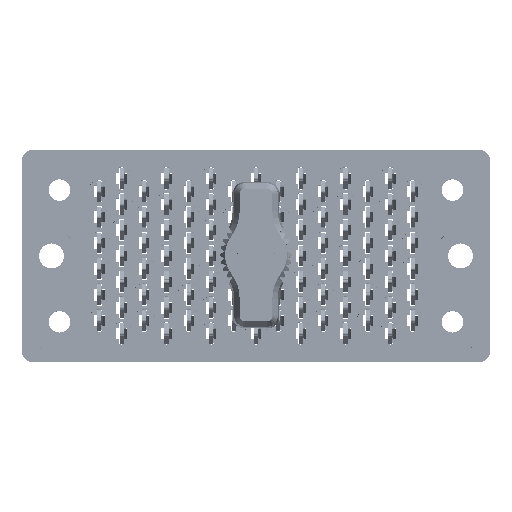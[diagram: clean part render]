
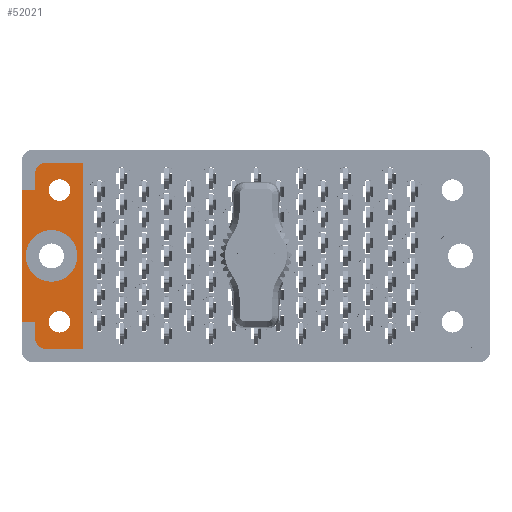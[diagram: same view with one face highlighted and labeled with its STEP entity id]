
A CAD part, top view. The second image highlights one B-rep face of the part: STEP entity #52021.
In plain terms, the highlighted planar face has unit normal (0, 0, 1).
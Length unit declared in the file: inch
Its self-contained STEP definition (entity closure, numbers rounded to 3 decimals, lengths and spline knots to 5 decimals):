
#267 = VECTOR ( 'NONE', #81808, 39.37008 ) ;
#488 = EDGE_CURVE ( 'NONE', #83931, #20014, #40906, .T. ) ;
#1366 = VERTEX_POINT ( 'NONE', #52308 ) ;
#2363 = AXIS2_PLACEMENT_3D ( 'NONE', #50024, #71200, #44172 ) ;
#2809 = ORIENTED_EDGE ( 'NONE', *, *, #488, .F. ) ;
#3448 = CARTESIAN_POINT ( 'NONE',  ( -1.1875, 0., -0.117 ) ) ;
#3648 = VERTEX_POINT ( 'NONE', #65361 ) ;
#3666 = EDGE_CURVE ( 'NONE', #20014, #83931, #4543, .T. ) ;
#4205 = ORIENTED_EDGE ( 'NONE', *, *, #11239, .F. ) ;
#4473 = EDGE_LOOP ( 'NONE', ( #41305, #84338, #61093, #54283, #52065, #55893, #63187, #67300, #24666, #56260 ) ) ;
#4543 = CIRCLE ( 'NONE', #33887, 0.0625 ) ;
#4942 = DIRECTION ( 'NONE',  ( 0., 0., 1. ) ) ;
#5032 = CIRCLE ( 'NONE', #50706, 0.062 ) ;
#5864 = CARTESIAN_POINT ( 'NONE',  ( -1.141, -0.3825, -0.117 ) ) ;
#6623 = EDGE_CURVE ( 'NONE', #80473, #18979, #70493, .T. ) ;
#7171 = CARTESIAN_POINT ( 'NONE',  ( -1.359, 0.617, -0.117 ) ) ;
#8485 = DIRECTION ( 'NONE',  ( 0., 0., 1. ) ) ;
#9338 = EDGE_CURVE ( 'NONE', #66660, #40700, #49050, .T. ) ;
#9568 = EDGE_CURVE ( 'NONE', #34214, #63157, #55380, .T. ) ;
#10014 = DIRECTION ( 'NONE',  ( 0., 0., 1. ) ) ;
#10477 = CARTESIAN_POINT ( 'NONE',  ( -1.2825, 0., -0.117 ) ) ;
#11239 = EDGE_CURVE ( 'NONE', #18979, #80473, #52926, .T. ) ;
#12429 = ORIENTED_EDGE ( 'NONE', *, *, #13034, .F. ) ;
#12678 = CARTESIAN_POINT ( 'NONE',  ( 0., -0.3825, -0.117 ) ) ;
#13034 = EDGE_CURVE ( 'NONE', #40700, #66660, #16687, .T. ) ;
#15766 = ORIENTED_EDGE ( 'NONE', *, *, #9338, .F. ) ;
#16687 = CIRCLE ( 'NONE', #18659, 0.0625 ) ;
#17314 = CARTESIAN_POINT ( 'NONE',  ( -1.005, 0.617, -0.117 ) ) ;
#17537 = CARTESIAN_POINT ( 'NONE',  ( -1.005, -0.54, -0.117 ) ) ;
#18172 = DIRECTION ( 'NONE',  ( 0., 1., 0. ) ) ;
#18659 = AXIS2_PLACEMENT_3D ( 'NONE', #79524, #4942, #59246 ) ;
#18979 = VERTEX_POINT ( 'NONE', #20722 ) ;
#19169 = DIRECTION ( 'NONE',  ( 0., -1., 0. ) ) ;
#19400 = EDGE_LOOP ( 'NONE', ( #2809, #85026 ) ) ;
#19715 = AXIS2_PLACEMENT_3D ( 'NONE', #71925, #45774, #79546 ) ;
#20014 = VERTEX_POINT ( 'NONE', #69586 ) ;
#20722 = CARTESIAN_POINT ( 'NONE',  ( -1.0375, 0., -0.117 ) ) ;
#21952 = CARTESIAN_POINT ( 'NONE',  ( -1.0785, -0.3825, -0.117 ) ) ;
#21995 = CARTESIAN_POINT ( 'NONE',  ( -1.359, -0.3825, -0.117 ) ) ;
#22975 = VERTEX_POINT ( 'NONE', #34861 ) ;
#23161 = VERTEX_POINT ( 'NONE', #64715 ) ;
#23983 = DIRECTION ( 'NONE',  ( 1., 0., 0. ) ) ;
#24666 = ORIENTED_EDGE ( 'NONE', *, *, #32924, .T. ) ;
#24702 = ORIENTED_EDGE ( 'NONE', *, *, #6623, .F. ) ;
#25692 = DIRECTION ( 'NONE',  ( 0., 0., 1. ) ) ;
#28446 = DIRECTION ( 'NONE',  ( 0., 0., 1. ) ) ;
#29346 = VECTOR ( 'NONE', #71869, 39.37008 ) ;
#29974 = CARTESIAN_POINT ( 'NONE',  ( -1.359, -0.617, -0.117 ) ) ;
#30174 = FACE_BOUND ( 'NONE', #85784, .T. ) ;
#31010 = DIRECTION ( 'NONE',  ( 0., 0., 1. ) ) ;
#32502 = CARTESIAN_POINT ( 'NONE',  ( 0., -0.54, -0.117 ) ) ;
#32924 = EDGE_CURVE ( 'NONE', #42397, #63157, #81279, .T. ) ;
#33373 = EDGE_CURVE ( 'NONE', #63286, #3648, #51752, .T. ) ;
#33613 = DIRECTION ( 'NONE',  ( 1., 0., 0. ) ) ;
#33887 = AXIS2_PLACEMENT_3D ( 'NONE', #59446, #25692, #33613 ) ;
#34214 = VERTEX_POINT ( 'NONE', #67780 ) ;
#34837 = CARTESIAN_POINT ( 'NONE',  ( 0., 0.3825, -0.117 ) ) ;
#34861 = CARTESIAN_POINT ( 'NONE',  ( -1.2825, 0.3825, -0.117 ) ) ;
#36032 = LINE ( 'NONE', #34837, #267 ) ;
#36096 = EDGE_CURVE ( 'NONE', #3648, #1366, #69596, .T. ) ;
#36127 = VECTOR ( 'NONE', #19169, 39.37008 ) ;
#37623 = AXIS2_PLACEMENT_3D ( 'NONE', #5864, #8485, #55420 ) ;
#38096 = EDGE_CURVE ( 'NONE', #59959, #22975, #82884, .T. ) ;
#40381 = CARTESIAN_POINT ( 'NONE',  ( -1.2825, 0., -0.117 ) ) ;
#40700 = VERTEX_POINT ( 'NONE', #72194 ) ;
#40901 = LINE ( 'NONE', #32502, #29346 ) ;
#40906 = CIRCLE ( 'NONE', #74804, 0.0625 ) ;
#41305 = ORIENTED_EDGE ( 'NONE', *, *, #86651, .T. ) ;
#42397 = VERTEX_POINT ( 'NONE', #57712 ) ;
#44172 = DIRECTION ( 'NONE',  ( 1., 0., 0. ) ) ;
#44466 = DIRECTION ( 'NONE',  ( 1., 0., 0. ) ) ;
#45774 = DIRECTION ( 'NONE',  ( 0., 0., 1. ) ) ;
#48933 = CIRCLE ( 'NONE', #2363, 0.062 ) ;
#49050 = CIRCLE ( 'NONE', #37623, 0.0625 ) ;
#50024 = CARTESIAN_POINT ( 'NONE',  ( -1.2205, 0.478, -0.117 ) ) ;
#50706 = AXIS2_PLACEMENT_3D ( 'NONE', #70081, #63293, #44466 ) ;
#50919 = EDGE_CURVE ( 'NONE', #63286, #23161, #40901, .T. ) ;
#51752 = LINE ( 'NONE', #17314, #71763 ) ;
#51805 = VECTOR ( 'NONE', #68301, 39.37008 ) ;
#52021 = ADVANCED_FACE ( 'NONE', ( #30174, #84902, #62801, #63805 ), #57251, .T. ) ;
#52065 = ORIENTED_EDGE ( 'NONE', *, *, #36096, .T. ) ;
#52308 = CARTESIAN_POINT ( 'NONE',  ( -1.2205, 0.54, -0.117 ) ) ;
#52926 = CIRCLE ( 'NONE', #19715, 0.15 ) ;
#53950 = DIRECTION ( 'NONE',  ( 1., 0., 0. ) ) ;
#54283 = ORIENTED_EDGE ( 'NONE', *, *, #33373, .T. ) ;
#55380 = LINE ( 'NONE', #12678, #71177 ) ;
#55420 = DIRECTION ( 'NONE',  ( 1., 0., 0. ) ) ;
#55742 = EDGE_CURVE ( 'NONE', #22975, #42397, #36032, .T. ) ;
#55893 = ORIENTED_EDGE ( 'NONE', *, *, #71725, .T. ) ;
#56260 = ORIENTED_EDGE ( 'NONE', *, *, #9568, .F. ) ;
#57251 = PLANE ( 'NONE',  #84667 ) ;
#57712 = CARTESIAN_POINT ( 'NONE',  ( -1.359, 0.3825, -0.117 ) ) ;
#58397 = VERTEX_POINT ( 'NONE', #61233 ) ;
#59246 = DIRECTION ( 'NONE',  ( 1., 0., 0. ) ) ;
#59446 = CARTESIAN_POINT ( 'NONE',  ( -1.141, 0.3825, -0.117 ) ) ;
#59807 = CARTESIAN_POINT ( 'NONE',  ( -1.2035, 0.3825, -0.117 ) ) ;
#59948 = DIRECTION ( 'NONE',  ( -1., 0., 0. ) ) ;
#59959 = VERTEX_POINT ( 'NONE', #69256 ) ;
#61093 = ORIENTED_EDGE ( 'NONE', *, *, #50919, .F. ) ;
#61113 = VECTOR ( 'NONE', #68319, 39.37008 ) ;
#61233 = CARTESIAN_POINT ( 'NONE',  ( -1.2825, -0.478, -0.117 ) ) ;
#62193 = AXIS2_PLACEMENT_3D ( 'NONE', #3448, #31010, #23983 ) ;
#62801 = FACE_BOUND ( 'NONE', #66374, .T. ) ;
#63157 = VERTEX_POINT ( 'NONE', #21995 ) ;
#63187 = ORIENTED_EDGE ( 'NONE', *, *, #38096, .T. ) ;
#63286 = VERTEX_POINT ( 'NONE', #17537 ) ;
#63293 = DIRECTION ( 'NONE',  ( 0., 0., 1. ) ) ;
#63805 = FACE_OUTER_BOUND ( 'NONE', #4473, .T. ) ;
#64715 = CARTESIAN_POINT ( 'NONE',  ( -1.2205, -0.54, -0.117 ) ) ;
#65005 = VECTOR ( 'NONE', #84201, 39.37008 ) ;
#65140 = CARTESIAN_POINT ( 'NONE',  ( -1.3375, 0., -0.117 ) ) ;
#65361 = CARTESIAN_POINT ( 'NONE',  ( -1.005, 0.54, -0.117 ) ) ;
#66374 = EDGE_LOOP ( 'NONE', ( #4205, #24702 ) ) ;
#66660 = VERTEX_POINT ( 'NONE', #21952 ) ;
#67300 = ORIENTED_EDGE ( 'NONE', *, *, #55742, .T. ) ;
#67780 = CARTESIAN_POINT ( 'NONE',  ( -1.2825, -0.3825, -0.117 ) ) ;
#68301 = DIRECTION ( 'NONE',  ( 0., -1., 0. ) ) ;
#68319 = DIRECTION ( 'NONE',  ( -1., 0., 0. ) ) ;
#68609 = CARTESIAN_POINT ( 'NONE',  ( 0., 0.54, -0.117 ) ) ;
#69256 = CARTESIAN_POINT ( 'NONE',  ( -1.2825, 0.478, -0.117 ) ) ;
#69586 = CARTESIAN_POINT ( 'NONE',  ( -1.0785, 0.3825, -0.117 ) ) ;
#69596 = LINE ( 'NONE', #68609, #61113 ) ;
#70081 = CARTESIAN_POINT ( 'NONE',  ( -1.2205, -0.478, -0.117 ) ) ;
#70249 = DIRECTION ( 'NONE',  ( 1., 0., 0. ) ) ;
#70493 = CIRCLE ( 'NONE', #62193, 0.15 ) ;
#71177 = VECTOR ( 'NONE', #59948, 39.37008 ) ;
#71200 = DIRECTION ( 'NONE',  ( 0., 0., 1. ) ) ;
#71725 = EDGE_CURVE ( 'NONE', #1366, #59959, #48933, .T. ) ;
#71763 = VECTOR ( 'NONE', #18172, 39.37008 ) ;
#71818 = LINE ( 'NONE', #40381, #51805 ) ;
#71869 = DIRECTION ( 'NONE',  ( -1., 0., 0. ) ) ;
#71925 = CARTESIAN_POINT ( 'NONE',  ( -1.1875, 0., -0.117 ) ) ;
#72194 = CARTESIAN_POINT ( 'NONE',  ( -1.2035, -0.3825, -0.117 ) ) ;
#74804 = AXIS2_PLACEMENT_3D ( 'NONE', #82176, #28446, #53950 ) ;
#79524 = CARTESIAN_POINT ( 'NONE',  ( -1.141, -0.3825, -0.117 ) ) ;
#79546 = DIRECTION ( 'NONE',  ( 1., 0., 0. ) ) ;
#80473 = VERTEX_POINT ( 'NONE', #65140 ) ;
#80963 = EDGE_CURVE ( 'NONE', #58397, #23161, #5032, .T. ) ;
#81279 = LINE ( 'NONE', #7171, #36127 ) ;
#81808 = DIRECTION ( 'NONE',  ( -1., 0., 0. ) ) ;
#82176 = CARTESIAN_POINT ( 'NONE',  ( -1.141, 0.3825, -0.117 ) ) ;
#82884 = LINE ( 'NONE', #10477, #65005 ) ;
#83931 = VERTEX_POINT ( 'NONE', #59807 ) ;
#84201 = DIRECTION ( 'NONE',  ( 0., -1., 0. ) ) ;
#84338 = ORIENTED_EDGE ( 'NONE', *, *, #80963, .T. ) ;
#84667 = AXIS2_PLACEMENT_3D ( 'NONE', #29974, #10014, #70249 ) ;
#84902 = FACE_BOUND ( 'NONE', #19400, .T. ) ;
#85026 = ORIENTED_EDGE ( 'NONE', *, *, #3666, .F. ) ;
#85784 = EDGE_LOOP ( 'NONE', ( #12429, #15766 ) ) ;
#86651 = EDGE_CURVE ( 'NONE', #34214, #58397, #71818, .T. ) ;
